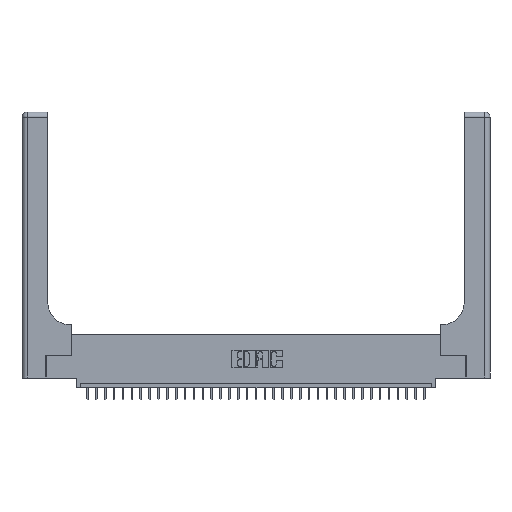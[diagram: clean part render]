
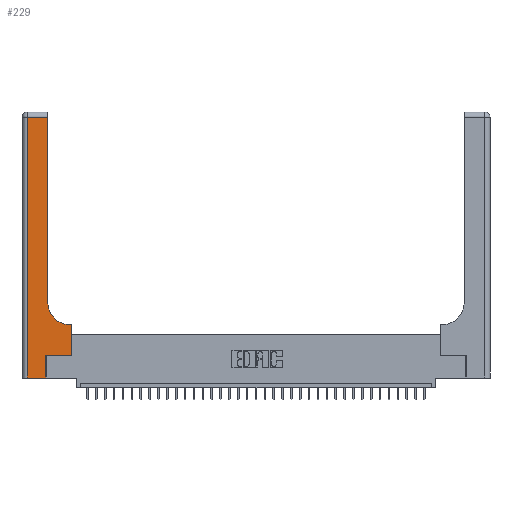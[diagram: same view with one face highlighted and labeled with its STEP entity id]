
A CAD part, top view. The second image highlights one B-rep face of the part: STEP entity #229.
In plain terms, the highlighted planar face has unit normal (0, 0, 1).
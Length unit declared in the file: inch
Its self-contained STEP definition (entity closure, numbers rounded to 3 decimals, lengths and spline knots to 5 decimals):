
#135 = CARTESIAN_POINT ( 'NONE',  ( 0.269, 0.25, 0.37 ) ) ;
#147 = EDGE_CURVE ( 'NONE', #17929, #4330, #2715, .T. ) ;
#171 = EDGE_CURVE ( 'NONE', #4330, #33484, #21557, .T. ) ;
#229 = ADVANCED_FACE ( 'NONE', ( #940 ), #22613, .F. ) ;
#940 = FACE_OUTER_BOUND ( 'NONE', #2586, .T. ) ;
#1748 = CARTESIAN_POINT ( 'NONE',  ( 0.06, 2.94, 0.37 ) ) ;
#1994 = AXIS2_PLACEMENT_3D ( 'NONE', #27428, #3245, #19786 ) ;
#2586 = EDGE_LOOP ( 'NONE', ( #26491, #21458, #7578, #14258, #26176, #25418, #11731, #6019, #19330 ) ) ;
#2588 = CARTESIAN_POINT ( 'NONE',  ( 0.5415, 0.85, 0.37 ) ) ;
#2715 = LINE ( 'NONE', #32242, #28649 ) ;
#2797 = CARTESIAN_POINT ( 'NONE',  ( 0.5415, 0.6, 0.37 ) ) ;
#3245 = DIRECTION ( 'NONE',  ( 0., 0., -1. ) ) ;
#3257 = VERTEX_POINT ( 'NONE', #26068 ) ;
#3570 = DIRECTION ( 'NONE',  ( 1., 0., 0. ) ) ;
#4330 = VERTEX_POINT ( 'NONE', #20276 ) ;
#4360 = EDGE_CURVE ( 'NONE', #25409, #26677, #9596, .T. ) ;
#5266 = LINE ( 'NONE', #29956, #33920 ) ;
#5326 = EDGE_CURVE ( 'NONE', #33484, #3257, #17471, .T. ) ;
#5432 = DIRECTION ( 'NONE',  ( 0., 0., -1. ) ) ;
#6019 = ORIENTED_EDGE ( 'NONE', *, *, #4360, .T. ) ;
#6698 = VECTOR ( 'NONE', #8763, 39.37008 ) ;
#7480 = AXIS2_PLACEMENT_3D ( 'NONE', #2588, #5432, #16312 ) ;
#7578 = ORIENTED_EDGE ( 'NONE', *, *, #24565, .T. ) ;
#8242 = VECTOR ( 'NONE', #3570, 39.37008 ) ;
#8763 = DIRECTION ( 'NONE',  ( 0., -1., 0. ) ) ;
#9110 = LINE ( 'NONE', #30616, #6698 ) ;
#9200 = VECTOR ( 'NONE', #20009, 39.37008 ) ;
#9596 = LINE ( 'NONE', #14418, #19586 ) ;
#10716 = DIRECTION ( 'NONE',  ( 0., 1., 0. ) ) ;
#11731 = ORIENTED_EDGE ( 'NONE', *, *, #23996, .T. ) ;
#11801 = LINE ( 'NONE', #33125, #20333 ) ;
#13471 = DIRECTION ( 'NONE',  ( 0., 1., 0. ) ) ;
#13558 = EDGE_CURVE ( 'NONE', #26677, #25723, #34714, .T. ) ;
#14258 = ORIENTED_EDGE ( 'NONE', *, *, #147, .T. ) ;
#14418 = CARTESIAN_POINT ( 'NONE',  ( 0.2915, 0.6, 0.37 ) ) ;
#16312 = DIRECTION ( 'NONE',  ( 1., 0., 0. ) ) ;
#17288 = CARTESIAN_POINT ( 'NONE',  ( 0.269, 0.25, 0.37 ) ) ;
#17441 = VERTEX_POINT ( 'NONE', #27024 ) ;
#17471 = LINE ( 'NONE', #17288, #8242 ) ;
#17542 = CARTESIAN_POINT ( 'NONE',  ( 0.2915, 3., 0.37 ) ) ;
#17792 = DIRECTION ( 'NONE',  ( -1., 0., 0. ) ) ;
#17929 = VERTEX_POINT ( 'NONE', #30669 ) ;
#19176 = CARTESIAN_POINT ( 'NONE',  ( 0.5585, 0.6, 0.37 ) ) ;
#19330 = ORIENTED_EDGE ( 'NONE', *, *, #13558, .T. ) ;
#19586 = VECTOR ( 'NONE', #17792, 39.37008 ) ;
#19786 = DIRECTION ( 'NONE',  ( -1., 0., 0. ) ) ;
#20009 = DIRECTION ( 'NONE',  ( 0., 1., 0. ) ) ;
#20276 = CARTESIAN_POINT ( 'NONE',  ( 0.269, 0., 0.37 ) ) ;
#20333 = VECTOR ( 'NONE', #22629, 39.37008 ) ;
#21458 = ORIENTED_EDGE ( 'NONE', *, *, #24581, .T. ) ;
#21557 = LINE ( 'NONE', #32577, #30347 ) ;
#22613 = PLANE ( 'NONE',  #1994 ) ;
#22629 = DIRECTION ( 'NONE',  ( -1., 0., 0. ) ) ;
#22829 = LINE ( 'NONE', #17542, #9200 ) ;
#23996 = EDGE_CURVE ( 'NONE', #3257, #25409, #5266, .T. ) ;
#24565 = EDGE_CURVE ( 'NONE', #25306, #17929, #9110, .T. ) ;
#24581 = EDGE_CURVE ( 'NONE', #17441, #25306, #11801, .T. ) ;
#25306 = VERTEX_POINT ( 'NONE', #1748 ) ;
#25409 = VERTEX_POINT ( 'NONE', #19176 ) ;
#25418 = ORIENTED_EDGE ( 'NONE', *, *, #5326, .T. ) ;
#25723 = VERTEX_POINT ( 'NONE', #31919 ) ;
#26068 = CARTESIAN_POINT ( 'NONE',  ( 0.5585, 0.25, 0.37 ) ) ;
#26176 = ORIENTED_EDGE ( 'NONE', *, *, #171, .T. ) ;
#26491 = ORIENTED_EDGE ( 'NONE', *, *, #28424, .T. ) ;
#26677 = VERTEX_POINT ( 'NONE', #2797 ) ;
#27024 = CARTESIAN_POINT ( 'NONE',  ( 0.2915, 2.94, 0.37 ) ) ;
#27428 = CARTESIAN_POINT ( 'NONE',  ( 0., 3., 0.37 ) ) ;
#28424 = EDGE_CURVE ( 'NONE', #25723, #17441, #22829, .T. ) ;
#28649 = VECTOR ( 'NONE', #29195, 39.37008 ) ;
#29195 = DIRECTION ( 'NONE',  ( 1., 0., 0. ) ) ;
#29956 = CARTESIAN_POINT ( 'NONE',  ( 0.5585, 0.25, 0.37 ) ) ;
#30347 = VECTOR ( 'NONE', #10716, 39.37008 ) ;
#30616 = CARTESIAN_POINT ( 'NONE',  ( 0.06, 3., 0.37 ) ) ;
#30669 = CARTESIAN_POINT ( 'NONE',  ( 0.06, 0., 0.37 ) ) ;
#31919 = CARTESIAN_POINT ( 'NONE',  ( 0.2915, 0.85, 0.37 ) ) ;
#32242 = CARTESIAN_POINT ( 'NONE',  ( 0., 0., 0.37 ) ) ;
#32577 = CARTESIAN_POINT ( 'NONE',  ( 0.269, 0., 0.37 ) ) ;
#33125 = CARTESIAN_POINT ( 'NONE',  ( 0., 2.94, 0.37 ) ) ;
#33484 = VERTEX_POINT ( 'NONE', #135 ) ;
#33920 = VECTOR ( 'NONE', #13471, 39.37008 ) ;
#34714 = CIRCLE ( 'NONE', #7480, 0.25 ) ;
